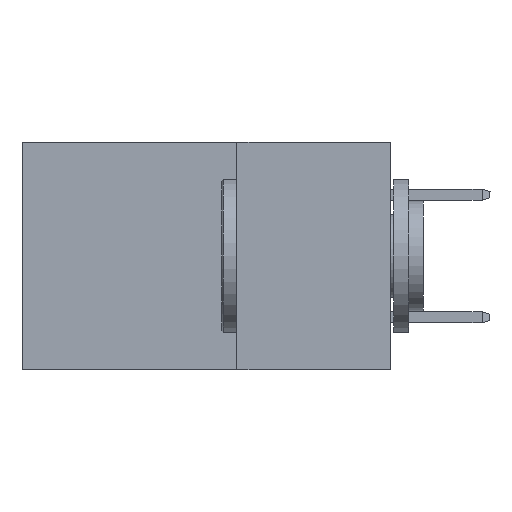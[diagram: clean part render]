
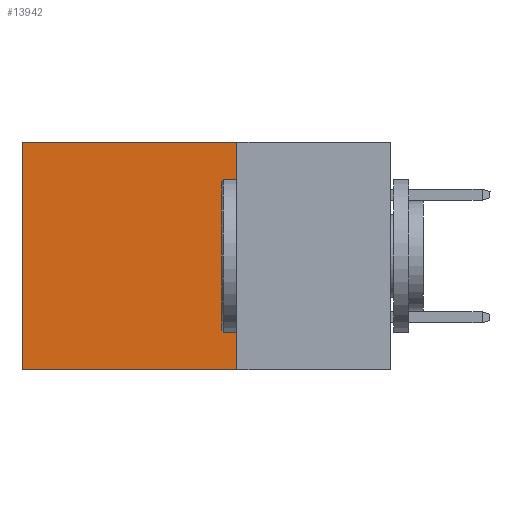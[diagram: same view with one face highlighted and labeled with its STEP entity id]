
A CAD part, left-side view. The second image highlights one B-rep face of the part: STEP entity #13942.
In plain terms, the highlighted planar face has unit normal (-1, 0, 0).
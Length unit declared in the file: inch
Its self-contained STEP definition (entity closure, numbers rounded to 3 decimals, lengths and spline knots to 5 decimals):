
#195 = ORIENTED_EDGE ( 'NONE', *, *, #42088, .F. ) ;
#2963 = VECTOR ( 'NONE', #5461, 39.37008 ) ;
#3196 = DIRECTION ( 'NONE',  ( 0., 0., -1. ) ) ;
#3205 = VERTEX_POINT ( 'NONE', #22691 ) ;
#4161 = VECTOR ( 'NONE', #21163, 39.37008 ) ;
#4192 = VECTOR ( 'NONE', #3196, 39.37008 ) ;
#5256 = EDGE_CURVE ( 'NONE', #36609, #15585, #40851, .T. ) ;
#5461 = DIRECTION ( 'NONE',  ( 0., 1., 0. ) ) ;
#6658 = CARTESIAN_POINT ( 'NONE',  ( 0.2875, 0.6, 0. ) ) ;
#8109 = ORIENTED_EDGE ( 'NONE', *, *, #16516, .T. ) ;
#10009 = CARTESIAN_POINT ( 'NONE',  ( 0.2875, 0.25, 0. ) ) ;
#11442 = VERTEX_POINT ( 'NONE', #18648 ) ;
#13294 = LINE ( 'NONE', #6658, #4192 ) ;
#13553 = CARTESIAN_POINT ( 'NONE',  ( 0.2875, 0.25, 0. ) ) ;
#13942 = ADVANCED_FACE ( 'NONE', ( #25450 ), #20271, .F. ) ;
#15585 = VERTEX_POINT ( 'NONE', #29018 ) ;
#16516 = EDGE_CURVE ( 'NONE', #3205, #11442, #13294, .T. ) ;
#17137 = ORIENTED_EDGE ( 'NONE', *, *, #5256, .F. ) ;
#18648 = CARTESIAN_POINT ( 'NONE',  ( 0.2875, 0.6, -0.37 ) ) ;
#20072 = LINE ( 'NONE', #29153, #36723 ) ;
#20271 = PLANE ( 'NONE',  #24356 ) ;
#21163 = DIRECTION ( 'NONE',  ( 0., 0., -1. ) ) ;
#22245 = CARTESIAN_POINT ( 'NONE',  ( 0.2875, 0.25, -0.37 ) ) ;
#22691 = CARTESIAN_POINT ( 'NONE',  ( 0.2875, 0.6, 0. ) ) ;
#23603 = DIRECTION ( 'NONE',  ( 0., 0., -1. ) ) ;
#24356 = AXIS2_PLACEMENT_3D ( 'NONE', #13553, #30964, #23603 ) ;
#25450 = FACE_OUTER_BOUND ( 'NONE', #32934, .T. ) ;
#29018 = CARTESIAN_POINT ( 'NONE',  ( 0.2875, 0.25, -0.37 ) ) ;
#29153 = CARTESIAN_POINT ( 'NONE',  ( 0.2875, 0.25, 0. ) ) ;
#30964 = DIRECTION ( 'NONE',  ( 1., 0., 0. ) ) ;
#32934 = EDGE_LOOP ( 'NONE', ( #8109, #195, #17137, #42734 ) ) ;
#35911 = DIRECTION ( 'NONE',  ( 0., 1., 0. ) ) ;
#36609 = VERTEX_POINT ( 'NONE', #10009 ) ;
#36723 = VECTOR ( 'NONE', #35911, 39.37008 ) ;
#37766 = CARTESIAN_POINT ( 'NONE',  ( 0.2875, 0.25, 0. ) ) ;
#38699 = LINE ( 'NONE', #22245, #2963 ) ;
#40851 = LINE ( 'NONE', #37766, #4161 ) ;
#40867 = EDGE_CURVE ( 'NONE', #36609, #3205, #20072, .T. ) ;
#42088 = EDGE_CURVE ( 'NONE', #15585, #11442, #38699, .T. ) ;
#42734 = ORIENTED_EDGE ( 'NONE', *, *, #40867, .T. ) ;
